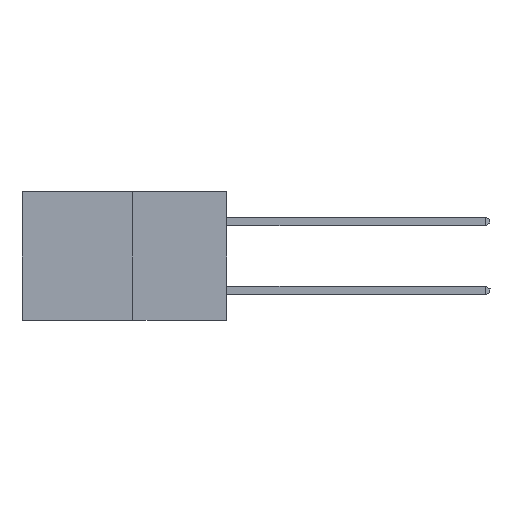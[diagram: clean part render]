
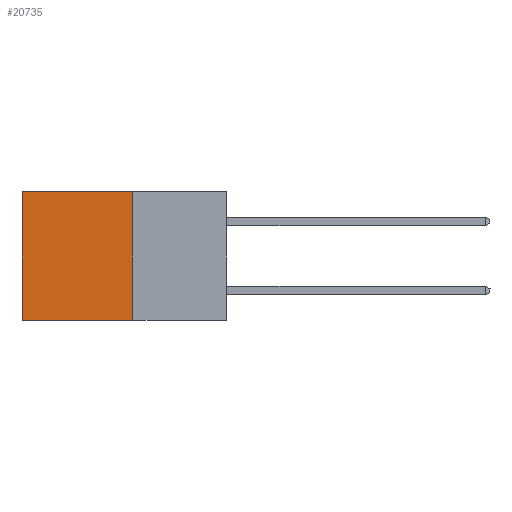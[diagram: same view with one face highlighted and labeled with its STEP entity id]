
A CAD part, left-side view. The second image highlights one B-rep face of the part: STEP entity #20735.
In plain terms, the highlighted planar face has unit normal (-1, 0, 0).
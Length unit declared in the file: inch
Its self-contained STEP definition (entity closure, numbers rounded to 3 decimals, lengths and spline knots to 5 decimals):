
#2768 = VECTOR ( 'NONE', #20977, 39.37008 ) ;
#3993 = EDGE_CURVE ( 'NONE', #27536, #6579, #16143, .T. ) ;
#4034 = EDGE_CURVE ( 'NONE', #4331, #27536, #26544, .T. ) ;
#4331 = VERTEX_POINT ( 'NONE', #5768 ) ;
#5768 = CARTESIAN_POINT ( 'NONE',  ( 0.277, 0.27, 0. ) ) ;
#6579 = VERTEX_POINT ( 'NONE', #8385 ) ;
#7436 = LINE ( 'NONE', #16757, #24455 ) ;
#7657 = CARTESIAN_POINT ( 'NONE',  ( 0.277, 0.27, 0. ) ) ;
#8385 = CARTESIAN_POINT ( 'NONE',  ( 0.277, 0.59, -0.37 ) ) ;
#9406 = ORIENTED_EDGE ( 'NONE', *, *, #24379, .F. ) ;
#12547 = FACE_OUTER_BOUND ( 'NONE', #13634, .T. ) ;
#12630 = EDGE_CURVE ( 'NONE', #4331, #18563, #27103, .T. ) ;
#12912 = DIRECTION ( 'NONE',  ( 0., 0., -1. ) ) ;
#13625 = ORIENTED_EDGE ( 'NONE', *, *, #4034, .T. ) ;
#13634 = EDGE_LOOP ( 'NONE', ( #17092, #9406, #28692, #13625 ) ) ;
#13891 = CARTESIAN_POINT ( 'NONE',  ( 0.277, 0.27, -0.37 ) ) ;
#14200 = CARTESIAN_POINT ( 'NONE',  ( 0.277, 0.59, -0.37 ) ) ;
#15439 = VECTOR ( 'NONE', #27456, 39.37008 ) ;
#16115 = DIRECTION ( 'NONE',  ( 0., 0., -1. ) ) ;
#16143 = LINE ( 'NONE', #14200, #15439 ) ;
#16757 = CARTESIAN_POINT ( 'NONE',  ( 0.277, 0.27, -0.37 ) ) ;
#17092 = ORIENTED_EDGE ( 'NONE', *, *, #3993, .T. ) ;
#17975 = CARTESIAN_POINT ( 'NONE',  ( 0.277, 0.27, -0.37 ) ) ;
#18563 = VERTEX_POINT ( 'NONE', #17975 ) ;
#18985 = DIRECTION ( 'NONE',  ( 0., 1., 0. ) ) ;
#19431 = AXIS2_PLACEMENT_3D ( 'NONE', #28288, #26186, #12912 ) ;
#19495 = PLANE ( 'NONE',  #19431 ) ;
#20735 = ADVANCED_FACE ( 'NONE', ( #12547 ), #19495, .F. ) ;
#20977 = DIRECTION ( 'NONE',  ( 0., 1., 0. ) ) ;
#24379 = EDGE_CURVE ( 'NONE', #18563, #6579, #7436, .T. ) ;
#24455 = VECTOR ( 'NONE', #18985, 39.37008 ) ;
#26186 = DIRECTION ( 'NONE',  ( 1., 0., 0. ) ) ;
#26200 = CARTESIAN_POINT ( 'NONE',  ( 0.277, 0.59, 0. ) ) ;
#26397 = VECTOR ( 'NONE', #16115, 39.37008 ) ;
#26544 = LINE ( 'NONE', #7657, #2768 ) ;
#27103 = LINE ( 'NONE', #13891, #26397 ) ;
#27456 = DIRECTION ( 'NONE',  ( 0., 0., -1. ) ) ;
#27536 = VERTEX_POINT ( 'NONE', #26200 ) ;
#28288 = CARTESIAN_POINT ( 'NONE',  ( 0.277, 0.27, -0.37 ) ) ;
#28692 = ORIENTED_EDGE ( 'NONE', *, *, #12630, .F. ) ;
